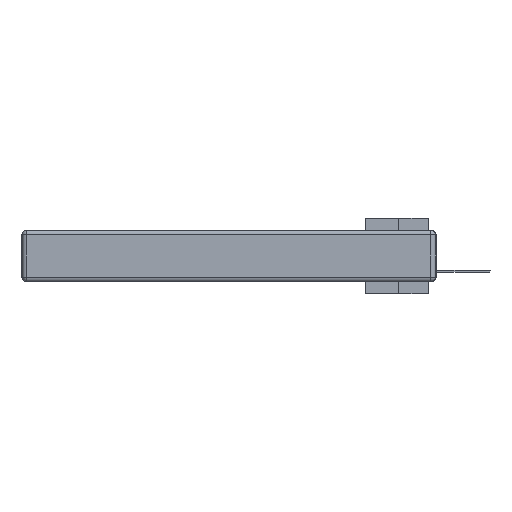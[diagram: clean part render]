
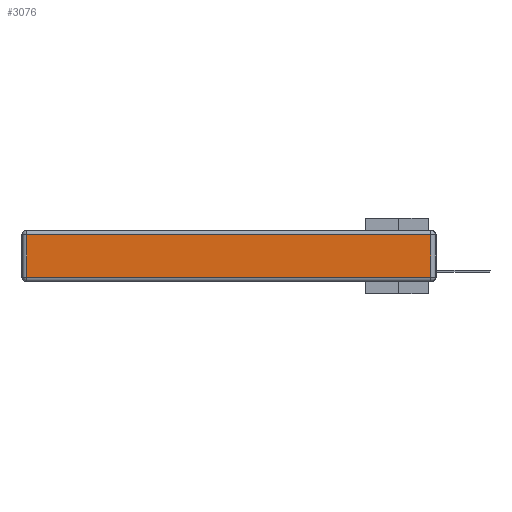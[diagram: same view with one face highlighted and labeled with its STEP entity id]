
A CAD part, left-side view. The second image highlights one B-rep face of the part: STEP entity #3076.
In plain terms, the highlighted planar face has unit normal (-1, 0, 0).
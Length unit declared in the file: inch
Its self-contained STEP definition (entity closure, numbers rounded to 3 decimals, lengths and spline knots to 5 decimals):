
#1927 = DIRECTION ( 'NONE',  ( 0., -1., 0. ) ) ;
#2548 = VECTOR ( 'NONE', #8902, 39.37008 ) ;
#2660 = EDGE_CURVE ( 'NONE', #11028, #23605, #5874, .T. ) ;
#3076 = ADVANCED_FACE ( 'NONE', ( #12254 ), #12626, .T. ) ;
#4426 = CARTESIAN_POINT ( 'NONE',  ( 0., 0., -0.313 ) ) ;
#5508 = LINE ( 'NONE', #37141, #10320 ) ;
#5874 = LINE ( 'NONE', #34692, #2548 ) ;
#6253 = ORIENTED_EDGE ( 'NONE', *, *, #36528, .T. ) ;
#7567 = VERTEX_POINT ( 'NONE', #22213 ) ;
#7585 = CARTESIAN_POINT ( 'NONE',  ( 0., 0.03, -0.313 ) ) ;
#7891 = AXIS2_PLACEMENT_3D ( 'NONE', #21120, #15288, #29573 ) ;
#8446 = VERTEX_POINT ( 'NONE', #7585 ) ;
#8902 = DIRECTION ( 'NONE',  ( 0., 1., 0. ) ) ;
#9399 = EDGE_CURVE ( 'NONE', #7567, #8446, #33603, .T. ) ;
#10320 = VECTOR ( 'NONE', #10990, 39.37008 ) ;
#10791 = CARTESIAN_POINT ( 'NONE',  ( 0., 0.03, -0.03 ) ) ;
#10990 = DIRECTION ( 'NONE',  ( 0., 0., -1. ) ) ;
#11028 = VERTEX_POINT ( 'NONE', #10791 ) ;
#12254 = FACE_OUTER_BOUND ( 'NONE', #30915, .T. ) ;
#12388 = DIRECTION ( 'NONE',  ( 0., 0., 1. ) ) ;
#12626 = PLANE ( 'NONE',  #7891 ) ;
#14487 = VECTOR ( 'NONE', #1927, 39.37008 ) ;
#15288 = DIRECTION ( 'NONE',  ( -1., 0., 0. ) ) ;
#19074 = ORIENTED_EDGE ( 'NONE', *, *, #32013, .T. ) ;
#19325 = ORIENTED_EDGE ( 'NONE', *, *, #9399, .T. ) ;
#19534 = CARTESIAN_POINT ( 'NONE',  ( 0., 2.72, -0.03 ) ) ;
#21120 = CARTESIAN_POINT ( 'NONE',  ( 0., 0., -0.343 ) ) ;
#22213 = CARTESIAN_POINT ( 'NONE',  ( 0., 2.72, -0.313 ) ) ;
#23605 = VERTEX_POINT ( 'NONE', #19534 ) ;
#24241 = LINE ( 'NONE', #26688, #24473 ) ;
#24473 = VECTOR ( 'NONE', #12388, 39.37008 ) ;
#26397 = ORIENTED_EDGE ( 'NONE', *, *, #2660, .T. ) ;
#26688 = CARTESIAN_POINT ( 'NONE',  ( 0., 0.03, -0.343 ) ) ;
#29573 = DIRECTION ( 'NONE',  ( 0., 0., 1. ) ) ;
#30915 = EDGE_LOOP ( 'NONE', ( #19325, #19074, #26397, #6253 ) ) ;
#32013 = EDGE_CURVE ( 'NONE', #8446, #11028, #24241, .T. ) ;
#33603 = LINE ( 'NONE', #4426, #14487 ) ;
#34692 = CARTESIAN_POINT ( 'NONE',  ( 0., 2.75, -0.03 ) ) ;
#36528 = EDGE_CURVE ( 'NONE', #23605, #7567, #5508, .T. ) ;
#37141 = CARTESIAN_POINT ( 'NONE',  ( 0., 2.72, -0.343 ) ) ;
